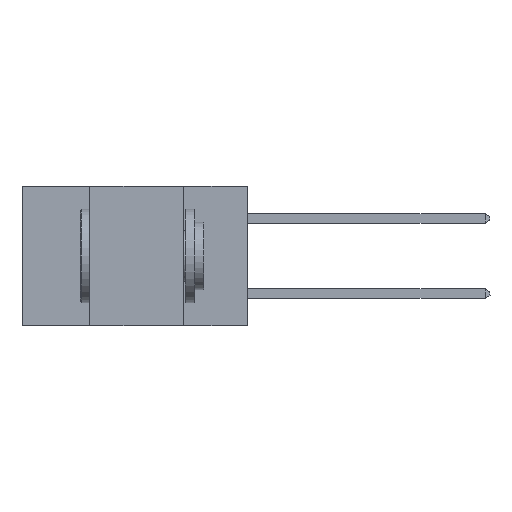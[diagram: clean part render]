
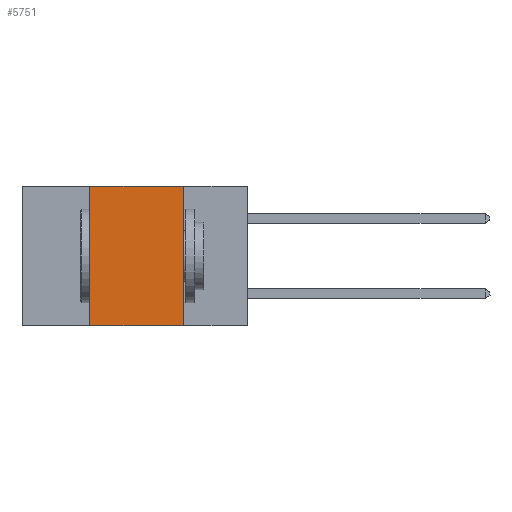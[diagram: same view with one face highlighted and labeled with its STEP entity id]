
A CAD part, left-side view. The second image highlights one B-rep face of the part: STEP entity #5751.
In plain terms, the highlighted planar face has unit normal (-1, 0, 0).
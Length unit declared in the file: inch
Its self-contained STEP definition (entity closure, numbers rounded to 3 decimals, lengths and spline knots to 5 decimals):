
#100 = CARTESIAN_POINT ( 'NONE',  ( 0., 0.6, -0.37 ) ) ;
#285 = ORIENTED_EDGE ( 'NONE', *, *, #7928, .F. ) ;
#422 = CARTESIAN_POINT ( 'NONE',  ( 0., 0.17, -0.37 ) ) ;
#504 = DIRECTION ( 'NONE',  ( 0., 0., -1. ) ) ;
#536 = DIRECTION ( 'NONE',  ( 0., -1., 0. ) ) ;
#1026 = FACE_OUTER_BOUND ( 'NONE', #7439, .T. ) ;
#1028 = DIRECTION ( 'NONE',  ( 0., -1., 0. ) ) ;
#1116 = ORIENTED_EDGE ( 'NONE', *, *, #8891, .F. ) ;
#1625 = VERTEX_POINT ( 'NONE', #4955 ) ;
#1944 = LINE ( 'NONE', #8971, #9129 ) ;
#2704 = DIRECTION ( 'NONE',  ( 0., 0., 1. ) ) ;
#3166 = LINE ( 'NONE', #100, #10508 ) ;
#3241 = CARTESIAN_POINT ( 'NONE',  ( 0., 0.6, 0. ) ) ;
#3938 = CARTESIAN_POINT ( 'NONE',  ( 0., 0.42, -0.37 ) ) ;
#4217 = LINE ( 'NONE', #5794, #6025 ) ;
#4578 = CARTESIAN_POINT ( 'NONE',  ( 0., 0.17, 0. ) ) ;
#4883 = PLANE ( 'NONE',  #9395 ) ;
#4955 = CARTESIAN_POINT ( 'NONE',  ( 0., 0.17, 0. ) ) ;
#5414 = LINE ( 'NONE', #4578, #6386 ) ;
#5609 = CARTESIAN_POINT ( 'NONE',  ( 0., 0.42, 0. ) ) ;
#5751 = ADVANCED_FACE ( 'NONE', ( #1026 ), #4883, .F. ) ;
#5762 = DIRECTION ( 'NONE',  ( 1., 0., 0. ) ) ;
#5794 = CARTESIAN_POINT ( 'NONE',  ( 0., 0.6, 0. ) ) ;
#6025 = VECTOR ( 'NONE', #536, 39.37008 ) ;
#6386 = VECTOR ( 'NONE', #9713, 39.37008 ) ;
#6416 = VERTEX_POINT ( 'NONE', #422 ) ;
#6496 = VERTEX_POINT ( 'NONE', #3938 ) ;
#7439 = EDGE_LOOP ( 'NONE', ( #285, #9804, #1116, #10600 ) ) ;
#7928 = EDGE_CURVE ( 'NONE', #1625, #6416, #5414, .T. ) ;
#8891 = EDGE_CURVE ( 'NONE', #6496, #9491, #1944, .T. ) ;
#8971 = CARTESIAN_POINT ( 'NONE',  ( 0., 0.42, 0. ) ) ;
#9129 = VECTOR ( 'NONE', #2704, 39.37008 ) ;
#9395 = AXIS2_PLACEMENT_3D ( 'NONE', #3241, #5762, #504 ) ;
#9491 = VERTEX_POINT ( 'NONE', #5609 ) ;
#9713 = DIRECTION ( 'NONE',  ( 0., 0., -1. ) ) ;
#9804 = ORIENTED_EDGE ( 'NONE', *, *, #10729, .F. ) ;
#10508 = VECTOR ( 'NONE', #1028, 39.37008 ) ;
#10600 = ORIENTED_EDGE ( 'NONE', *, *, #11112, .T. ) ;
#10729 = EDGE_CURVE ( 'NONE', #9491, #1625, #4217, .T. ) ;
#11112 = EDGE_CURVE ( 'NONE', #6496, #6416, #3166, .T. ) ;
